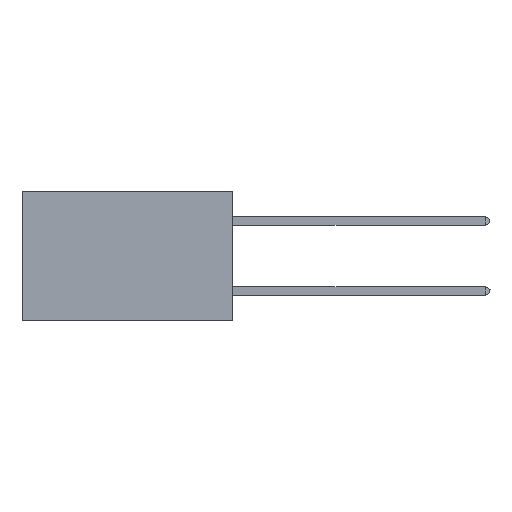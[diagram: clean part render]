
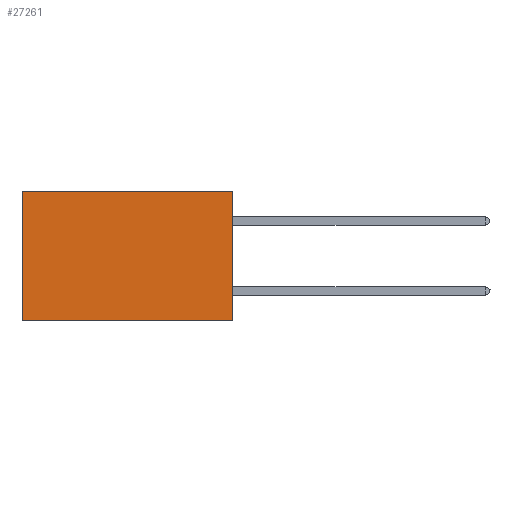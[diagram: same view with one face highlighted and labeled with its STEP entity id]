
A CAD part, left-side view. The second image highlights one B-rep face of the part: STEP entity #27261.
In plain terms, the highlighted planar face has unit normal (-1, 0, 0).
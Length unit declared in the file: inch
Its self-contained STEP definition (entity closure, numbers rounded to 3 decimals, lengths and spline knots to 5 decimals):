
#1049 = EDGE_CURVE ( 'NONE', #4935, #38348, #17241, .T. ) ;
#1694 = CARTESIAN_POINT ( 'NONE',  ( 0.2875, 0., 0. ) ) ;
#1721 = DIRECTION ( 'NONE',  ( 1., 0., 0. ) ) ;
#2170 = AXIS2_PLACEMENT_3D ( 'NONE', #26556, #1721, #17297 ) ;
#2819 = FACE_OUTER_BOUND ( 'NONE', #9545, .T. ) ;
#2853 = LINE ( 'NONE', #33693, #33496 ) ;
#3125 = CARTESIAN_POINT ( 'NONE',  ( 0.2875, 0.6, 0. ) ) ;
#3868 = VERTEX_POINT ( 'NONE', #3125 ) ;
#4935 = VERTEX_POINT ( 'NONE', #21593 ) ;
#6474 = EDGE_CURVE ( 'NONE', #3868, #38348, #33904, .T. ) ;
#7157 = CARTESIAN_POINT ( 'NONE',  ( 0.2875, 0., -0.37 ) ) ;
#8690 = PLANE ( 'NONE',  #2170 ) ;
#8970 = CARTESIAN_POINT ( 'NONE',  ( 0.2875, 0., 0. ) ) ;
#9545 = EDGE_LOOP ( 'NONE', ( #35585, #30234, #34928, #13491 ) ) ;
#11482 = CARTESIAN_POINT ( 'NONE',  ( 0.2875, 0.6, 0. ) ) ;
#13491 = ORIENTED_EDGE ( 'NONE', *, *, #23208, .T. ) ;
#17241 = LINE ( 'NONE', #7157, #23526 ) ;
#17297 = DIRECTION ( 'NONE',  ( 0., 0., -1. ) ) ;
#17741 = DIRECTION ( 'NONE',  ( 0., 1., 0. ) ) ;
#21593 = CARTESIAN_POINT ( 'NONE',  ( 0.2875, 0., -0.37 ) ) ;
#23208 = EDGE_CURVE ( 'NONE', #24380, #3868, #2853, .T. ) ;
#23526 = VECTOR ( 'NONE', #28953, 39.37008 ) ;
#24380 = VERTEX_POINT ( 'NONE', #8970 ) ;
#25591 = VECTOR ( 'NONE', #26053, 39.37008 ) ;
#26053 = DIRECTION ( 'NONE',  ( 0., 0., -1. ) ) ;
#26556 = CARTESIAN_POINT ( 'NONE',  ( 0.2875, 0., 0. ) ) ;
#26665 = DIRECTION ( 'NONE',  ( 0., 0., -1. ) ) ;
#27261 = ADVANCED_FACE ( 'NONE', ( #2819 ), #8690, .F. ) ;
#28013 = EDGE_CURVE ( 'NONE', #24380, #4935, #29016, .T. ) ;
#28953 = DIRECTION ( 'NONE',  ( 0., 1., 0. ) ) ;
#29016 = LINE ( 'NONE', #1694, #33879 ) ;
#30234 = ORIENTED_EDGE ( 'NONE', *, *, #1049, .F. ) ;
#33496 = VECTOR ( 'NONE', #17741, 39.37008 ) ;
#33693 = CARTESIAN_POINT ( 'NONE',  ( 0.2875, 0., 0. ) ) ;
#33879 = VECTOR ( 'NONE', #26665, 39.37008 ) ;
#33904 = LINE ( 'NONE', #11482, #25591 ) ;
#34639 = CARTESIAN_POINT ( 'NONE',  ( 0.2875, 0.6, -0.37 ) ) ;
#34928 = ORIENTED_EDGE ( 'NONE', *, *, #28013, .F. ) ;
#35585 = ORIENTED_EDGE ( 'NONE', *, *, #6474, .T. ) ;
#38348 = VERTEX_POINT ( 'NONE', #34639 ) ;
